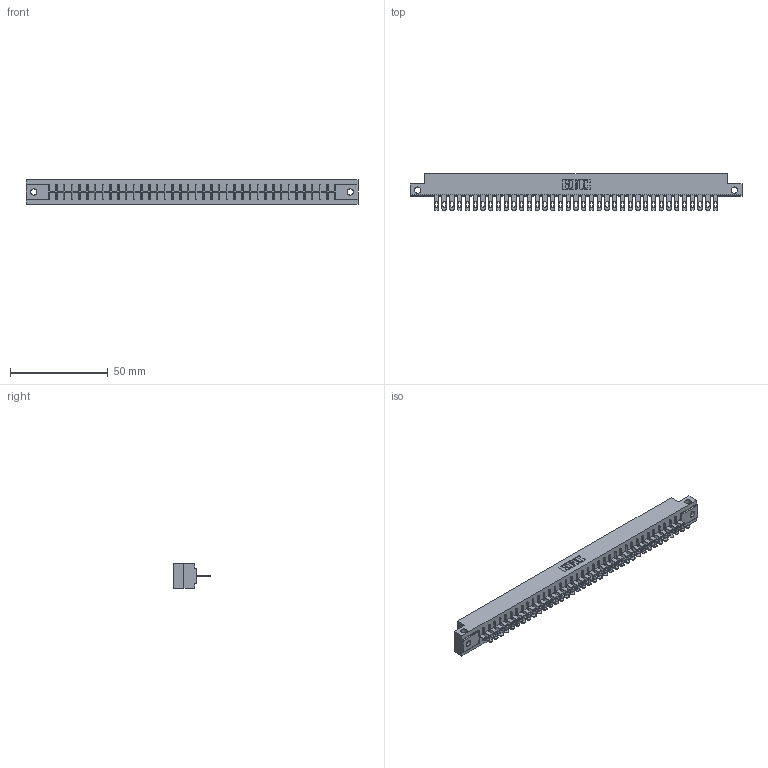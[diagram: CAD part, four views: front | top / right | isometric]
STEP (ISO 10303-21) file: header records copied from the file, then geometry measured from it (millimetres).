
FILE_DESCRIPTION (( 'STEP AP203' ), '1' );
FILE_NAME ('316-037-500-112.STEP', '2020-09-20T21:28:28', ( '' ), ( '' ), 'SwSTEP 2.0', 'SolidWorks 2020', '' );
FILE_SCHEMA (( 'CONFIG_CONTROL_DESIGN' ));
Length unit declared in the file: inch
Products named in the file (3): 306 Part_.128 Dia; 316-037-500-112; 306-290-001_100
Assembly tree (38 placements, depth 2):
  316-037-500-112
    306 Part_.128 Dia
    306-290-001_100  x37
Bounding box: 169.62 x 18.87 x 12.7 mm (x, y, z)
Volume: 18636.8 mm3; surface area: 19749.3 mm2
Topology: 38 solids, 38 shells, 2940 faces, 8307 edges, 5334 vertices
Faces by surface type: plane 1918, cylinder 874, sphere 148
Entity records: 35722 total; most frequent: CARTESIAN_POINT 6046, ORIENTED_EDGE 5950, DIRECTION 5901, EDGE_CURVE 2975, LINE 2307, VECTOR 2307, VERTEX_POINT 1878, AXIS2_PLACEMENT_3D 1797
